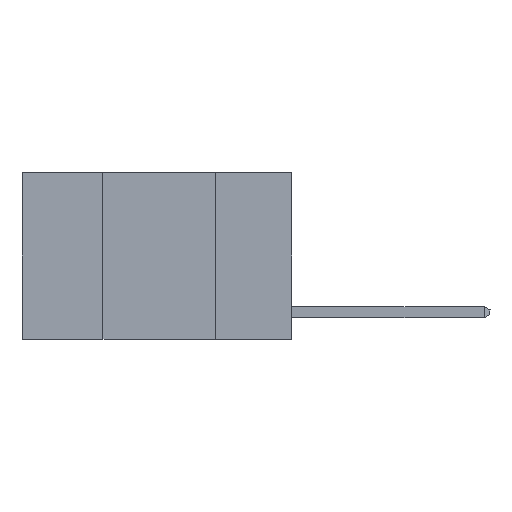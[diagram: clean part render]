
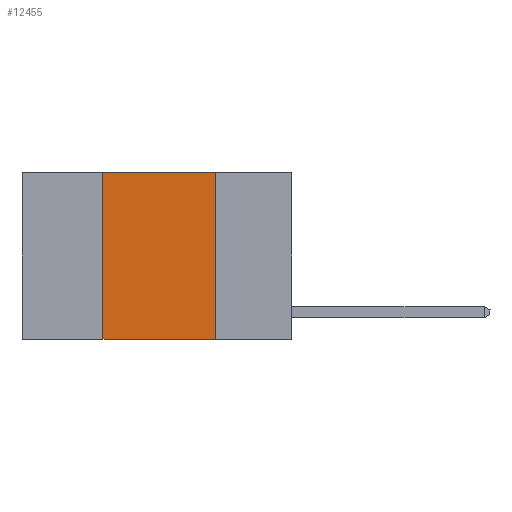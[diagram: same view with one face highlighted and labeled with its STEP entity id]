
A CAD part, left-side view. The second image highlights one B-rep face of the part: STEP entity #12455.
In plain terms, the highlighted planar face has unit normal (-1, 0, 0).
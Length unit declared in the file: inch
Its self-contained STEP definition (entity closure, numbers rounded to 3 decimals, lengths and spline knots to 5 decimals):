
#1874 = CARTESIAN_POINT ( 'NONE',  ( 0., 0.6, -0.37 ) ) ;
#1952 = EDGE_CURVE ( 'NONE', #8942, #15198, #15464, .T. ) ;
#1964 = VECTOR ( 'NONE', #10793, 39.37008 ) ;
#2187 = CARTESIAN_POINT ( 'NONE',  ( 0., 0.42, 0. ) ) ;
#3423 = DIRECTION ( 'NONE',  ( 0., 0., -1. ) ) ;
#3592 = ORIENTED_EDGE ( 'NONE', *, *, #12476, .T. ) ;
#3693 = CARTESIAN_POINT ( 'NONE',  ( 0., 0.17, 0. ) ) ;
#4252 = EDGE_CURVE ( 'NONE', #20539, #8942, #11533, .T. ) ;
#4906 = VECTOR ( 'NONE', #16009, 39.37008 ) ;
#4945 = LINE ( 'NONE', #3693, #12015 ) ;
#7120 = PLANE ( 'NONE',  #15085 ) ;
#7258 = VECTOR ( 'NONE', #12877, 39.37008 ) ;
#7289 = DIRECTION ( 'NONE',  ( 0., 0., -1. ) ) ;
#7997 = CARTESIAN_POINT ( 'NONE',  ( 0., 0.17, -0.37 ) ) ;
#8942 = VERTEX_POINT ( 'NONE', #2187 ) ;
#9580 = ORIENTED_EDGE ( 'NONE', *, *, #4252, .F. ) ;
#10531 = FACE_OUTER_BOUND ( 'NONE', #17321, .T. ) ;
#10597 = CARTESIAN_POINT ( 'NONE',  ( 0., 0.6, 0. ) ) ;
#10793 = DIRECTION ( 'NONE',  ( 0., 0., 1. ) ) ;
#11143 = CARTESIAN_POINT ( 'NONE',  ( 0., 0.6, 0. ) ) ;
#11471 = VERTEX_POINT ( 'NONE', #7997 ) ;
#11533 = LINE ( 'NONE', #12690, #1964 ) ;
#11663 = ORIENTED_EDGE ( 'NONE', *, *, #1952, .F. ) ;
#12015 = VECTOR ( 'NONE', #7289, 39.37008 ) ;
#12455 = ADVANCED_FACE ( 'NONE', ( #10531 ), #7120, .F. ) ;
#12476 = EDGE_CURVE ( 'NONE', #20539, #11471, #12801, .T. ) ;
#12690 = CARTESIAN_POINT ( 'NONE',  ( 0., 0.42, 0. ) ) ;
#12801 = LINE ( 'NONE', #1874, #4906 ) ;
#12877 = DIRECTION ( 'NONE',  ( 0., -1., 0. ) ) ;
#15085 = AXIS2_PLACEMENT_3D ( 'NONE', #10597, #19787, #3423 ) ;
#15198 = VERTEX_POINT ( 'NONE', #22838 ) ;
#15464 = LINE ( 'NONE', #11143, #7258 ) ;
#16009 = DIRECTION ( 'NONE',  ( 0., -1., 0. ) ) ;
#16546 = EDGE_CURVE ( 'NONE', #15198, #11471, #4945, .T. ) ;
#17321 = EDGE_LOOP ( 'NONE', ( #22384, #11663, #9580, #3592 ) ) ;
#19787 = DIRECTION ( 'NONE',  ( 1., 0., 0. ) ) ;
#20539 = VERTEX_POINT ( 'NONE', #21171 ) ;
#21171 = CARTESIAN_POINT ( 'NONE',  ( 0., 0.42, -0.37 ) ) ;
#22384 = ORIENTED_EDGE ( 'NONE', *, *, #16546, .F. ) ;
#22838 = CARTESIAN_POINT ( 'NONE',  ( 0., 0.17, 0. ) ) ;
